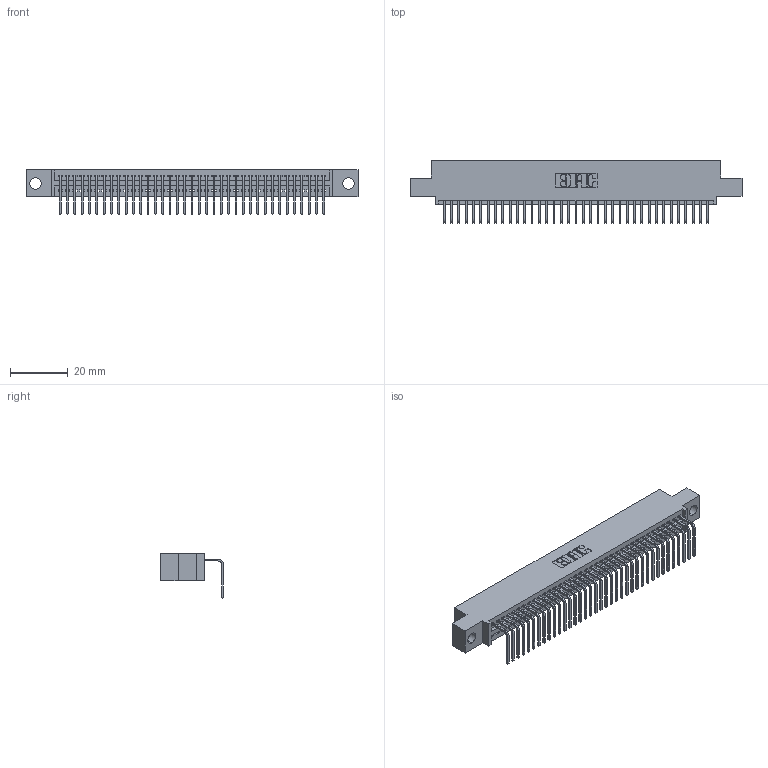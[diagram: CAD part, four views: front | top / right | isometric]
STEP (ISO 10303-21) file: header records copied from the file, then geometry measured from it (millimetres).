
FILE_DESCRIPTION (( 'STEP AP203' ), '1' );
FILE_NAME ('345-037-558-404.STEP', '2021-06-09T16:37:16', ( '' ), ( '' ), 'SwSTEP 2.0', 'SolidWorks 2020', '' );
FILE_SCHEMA (( 'CONFIG_CONTROL_DESIGN' ));
Length unit declared in the file: inch
Products named in the file (3): 345-292-001_558 Tail - 2; 345 Part_0.110 Offset - 0.156 Dia-TI; 345-037-558-404
Assembly tree (38 placements, depth 2):
  345-037-558-404
    345 Part_0.110 Offset - 0.156 Dia-TI
    345-292-001_558 Tail - 2  x37
Bounding box: 115.19 x 21.83 x 15.37 mm (x, y, z)
Volume: 10843.8 mm3; surface area: 14991.2 mm2
Topology: 38 solids, 38 shells, 2364 faces, 7123 edges, 4698 vertices
Faces by surface type: plane 1652, cylinder 712
Entity records: 29155 total; most frequent: CARTESIAN_POINT 5061, ORIENTED_EDGE 5030, DIRECTION 4425, EDGE_CURVE 2515, LINE 2235, VECTOR 2235, VERTEX_POINT 1674, AXIS2_PLACEMENT_3D 1095
